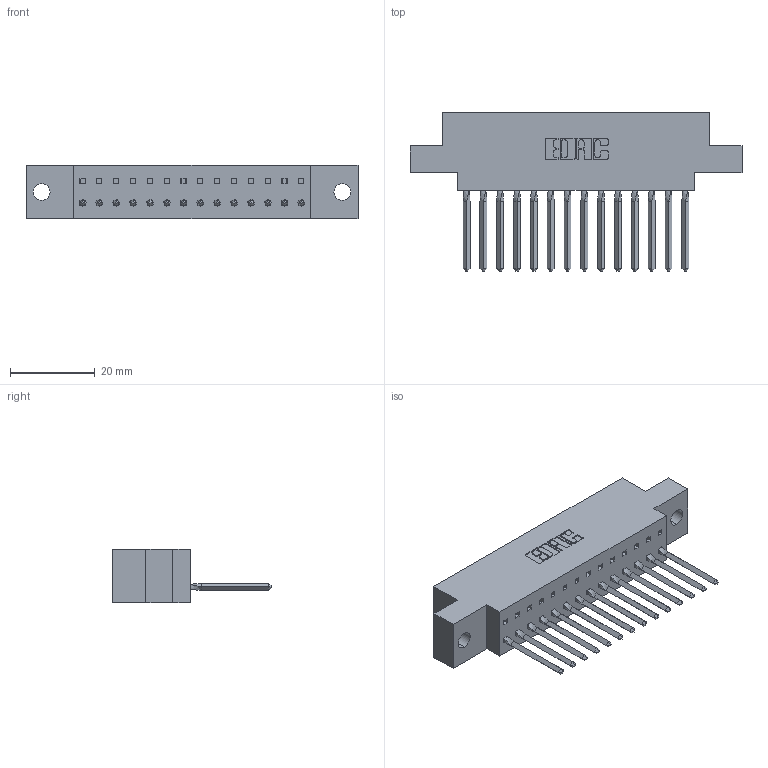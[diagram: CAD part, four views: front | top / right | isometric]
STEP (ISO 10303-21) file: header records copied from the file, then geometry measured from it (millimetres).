
FILE_DESCRIPTION (( 'STEP AP203' ), '1' );
FILE_NAME ('317-014-541-604.STEP', '2020-02-27T14:37:16', ( '' ), ( '' ), 'SwSTEP 2.0', 'SolidWorks 2016', '' );
FILE_SCHEMA (( 'CONFIG_CONTROL_DESIGN' ));
Length unit declared in the file: inch
Products named in the file (3): 317-290-002_541; 317-014-541-604; 317 Part_.156 Dia - TH
Assembly tree (15 placements, depth 2):
  317-014-541-604
    317 Part_.156 Dia - TH
    317-290-002_541  x14
Bounding box: 78.18 x 37.34 x 12.7 mm (x, y, z)
Volume: 11729.6 mm3; surface area: 15459.1 mm2
Topology: 15 solids, 15 shells, 2230 faces, 6351 edges, 4130 vertices
Faces by surface type: plane 1794, cylinder 380, bspline 56
Entity records: 25246 total; most frequent: CARTESIAN_POINT 5115, ORIENTED_EDGE 4382, DIRECTION 3579, EDGE_CURVE 2191, LINE 1827, VECTOR 1827, VERTEX_POINT 1452, AXIS2_PLACEMENT_3D 876
